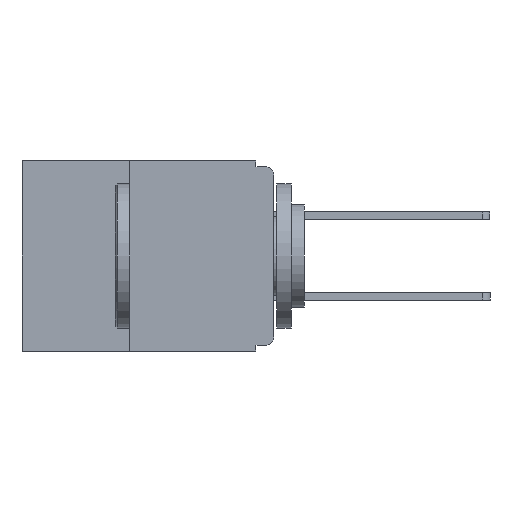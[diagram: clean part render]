
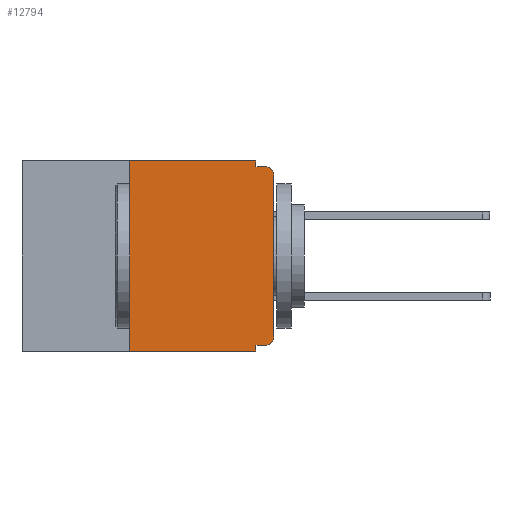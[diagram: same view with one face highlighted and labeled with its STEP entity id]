
A CAD part, left-side view. The second image highlights one B-rep face of the part: STEP entity #12794.
In plain terms, the highlighted planar face has unit normal (-1, 0, 0).
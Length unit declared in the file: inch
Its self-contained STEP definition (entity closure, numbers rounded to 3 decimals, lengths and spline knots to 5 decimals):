
#298 = DIRECTION ( 'NONE',  ( 0., 1., 0. ) ) ;
#384 = DIRECTION ( 'NONE',  ( 0., 0., -1. ) ) ;
#423 = ORIENTED_EDGE ( 'NONE', *, *, #16707, .F. ) ;
#598 = CARTESIAN_POINT ( 'NONE',  ( 0., 0.25, -0.33 ) ) ;
#791 = DIRECTION ( 'NONE',  ( 0., 0., 1. ) ) ;
#1061 = LINE ( 'NONE', #6859, #5854 ) ;
#1530 = ORIENTED_EDGE ( 'NONE', *, *, #5502, .F. ) ;
#1548 = EDGE_CURVE ( 'NONE', #3851, #9073, #20003, .T. ) ;
#1618 = DIRECTION ( 'NONE',  ( 0., 0., 1. ) ) ;
#1698 = CARTESIAN_POINT ( 'NONE',  ( 0., 0.031, 0. ) ) ;
#2040 = CARTESIAN_POINT ( 'NONE',  ( 0., 0., -0.32 ) ) ;
#2406 = ORIENTED_EDGE ( 'NONE', *, *, #16976, .F. ) ;
#2468 = EDGE_CURVE ( 'NONE', #5348, #15666, #21885, .T. ) ;
#3175 = CARTESIAN_POINT ( 'NONE',  ( 0., 0.25, 0. ) ) ;
#3291 = VERTEX_POINT ( 'NONE', #16460 ) ;
#3694 = LINE ( 'NONE', #22372, #10378 ) ;
#3746 = DIRECTION ( 'NONE',  ( 0., -1., 0. ) ) ;
#3851 = VERTEX_POINT ( 'NONE', #5782 ) ;
#3961 = EDGE_CURVE ( 'NONE', #15666, #5482, #3694, .T. ) ;
#4403 = CARTESIAN_POINT ( 'NONE',  ( 0., 0.015, -0.025 ) ) ;
#4457 = LINE ( 'NONE', #15519, #17992 ) ;
#4884 = EDGE_CURVE ( 'NONE', #3291, #14059, #13873, .T. ) ;
#4890 = ORIENTED_EDGE ( 'NONE', *, *, #1548, .T. ) ;
#4951 = DIRECTION ( 'NONE',  ( 0., 0., -1. ) ) ;
#5183 = ORIENTED_EDGE ( 'NONE', *, *, #2468, .F. ) ;
#5348 = VERTEX_POINT ( 'NONE', #13063 ) ;
#5482 = VERTEX_POINT ( 'NONE', #7385 ) ;
#5502 = EDGE_CURVE ( 'NONE', #14059, #5348, #1061, .T. ) ;
#5782 = CARTESIAN_POINT ( 'NONE',  ( 0., 0., -0.305 ) ) ;
#5854 = VECTOR ( 'NONE', #6908, 39.37008 ) ;
#5918 = EDGE_CURVE ( 'NONE', #17478, #3851, #20400, .T. ) ;
#6221 = DIRECTION ( 'NONE',  ( 0., 0., -1. ) ) ;
#6545 = VECTOR ( 'NONE', #1618, 39.37008 ) ;
#6859 = CARTESIAN_POINT ( 'NONE',  ( 0., 0.437, 0. ) ) ;
#6885 = ORIENTED_EDGE ( 'NONE', *, *, #4884, .F. ) ;
#6908 = DIRECTION ( 'NONE',  ( 0., -1., 0. ) ) ;
#7280 = VECTOR ( 'NONE', #298, 39.37008 ) ;
#7385 = CARTESIAN_POINT ( 'NONE',  ( 0., 0.015, -0.01 ) ) ;
#8467 = LINE ( 'NONE', #14328, #17801 ) ;
#8469 = DIRECTION ( 'NONE',  ( 0., 0., -1. ) ) ;
#9073 = VERTEX_POINT ( 'NONE', #19768 ) ;
#9863 = AXIS2_PLACEMENT_3D ( 'NONE', #20633, #18973, #8469 ) ;
#9920 = EDGE_LOOP ( 'NONE', ( #4890, #15395, #18150, #5183, #1530, #6885, #22184, #423, #2406, #12957 ) ) ;
#10378 = VECTOR ( 'NONE', #22081, 39.37008 ) ;
#10852 = EDGE_CURVE ( 'NONE', #3291, #18784, #8467, .T. ) ;
#12794 = ADVANCED_FACE ( 'NONE', ( #21772 ), #22323, .F. ) ;
#12957 = ORIENTED_EDGE ( 'NONE', *, *, #5918, .T. ) ;
#13063 = CARTESIAN_POINT ( 'NONE',  ( 0., 0.031, 0. ) ) ;
#13873 = LINE ( 'NONE', #598, #18002 ) ;
#14059 = VERTEX_POINT ( 'NONE', #3175 ) ;
#14172 = CARTESIAN_POINT ( 'NONE',  ( 0., 0.031, -0.01 ) ) ;
#14328 = CARTESIAN_POINT ( 'NONE',  ( 0., 0.437, -0.33 ) ) ;
#14999 = VERTEX_POINT ( 'NONE', #19332 ) ;
#15395 = ORIENTED_EDGE ( 'NONE', *, *, #21621, .T. ) ;
#15429 = DIRECTION ( 'NONE',  ( 0., 0., -1. ) ) ;
#15458 = CARTESIAN_POINT ( 'NONE',  ( 0., 0.015, -0.305 ) ) ;
#15476 = DIRECTION ( 'NONE',  ( -1., 0., 0. ) ) ;
#15519 = CARTESIAN_POINT ( 'NONE',  ( 0., 0.031, -0.33 ) ) ;
#15623 = AXIS2_PLACEMENT_3D ( 'NONE', #15458, #15476, #15429 ) ;
#15666 = VERTEX_POINT ( 'NONE', #14172 ) ;
#16460 = CARTESIAN_POINT ( 'NONE',  ( 0., 0.25, -0.33 ) ) ;
#16606 = LINE ( 'NONE', #2040, #7280 ) ;
#16707 = EDGE_CURVE ( 'NONE', #14999, #18784, #4457, .T. ) ;
#16761 = DIRECTION ( 'NONE',  ( -1., 0., 0. ) ) ;
#16976 = EDGE_CURVE ( 'NONE', #17478, #14999, #16606, .T. ) ;
#17297 = VECTOR ( 'NONE', #384, 39.37008 ) ;
#17478 = VERTEX_POINT ( 'NONE', #18414 ) ;
#17801 = VECTOR ( 'NONE', #3746, 39.37008 ) ;
#17992 = VECTOR ( 'NONE', #4951, 39.37008 ) ;
#18002 = VECTOR ( 'NONE', #791, 39.37008 ) ;
#18150 = ORIENTED_EDGE ( 'NONE', *, *, #3961, .F. ) ;
#18414 = CARTESIAN_POINT ( 'NONE',  ( 0., 0.015, -0.32 ) ) ;
#18784 = VERTEX_POINT ( 'NONE', #22023 ) ;
#18973 = DIRECTION ( 'NONE',  ( 1., 0., 0. ) ) ;
#19332 = CARTESIAN_POINT ( 'NONE',  ( 0., 0.031, -0.32 ) ) ;
#19398 = AXIS2_PLACEMENT_3D ( 'NONE', #4403, #16761, #6221 ) ;
#19768 = CARTESIAN_POINT ( 'NONE',  ( 0., 0., -0.025 ) ) ;
#19773 = CARTESIAN_POINT ( 'NONE',  ( 0., 0., 0. ) ) ;
#20003 = LINE ( 'NONE', #19773, #6545 ) ;
#20400 = CIRCLE ( 'NONE', #15623, 0.015 ) ;
#20633 = CARTESIAN_POINT ( 'NONE',  ( 0., 0.437, 0. ) ) ;
#21621 = EDGE_CURVE ( 'NONE', #9073, #5482, #21835, .T. ) ;
#21772 = FACE_OUTER_BOUND ( 'NONE', #9920, .T. ) ;
#21835 = CIRCLE ( 'NONE', #19398, 0.015 ) ;
#21885 = LINE ( 'NONE', #1698, #17297 ) ;
#22023 = CARTESIAN_POINT ( 'NONE',  ( 0., 0.031, -0.33 ) ) ;
#22081 = DIRECTION ( 'NONE',  ( 0., -1., 0. ) ) ;
#22184 = ORIENTED_EDGE ( 'NONE', *, *, #10852, .T. ) ;
#22323 = PLANE ( 'NONE',  #9863 ) ;
#22372 = CARTESIAN_POINT ( 'NONE',  ( 0., 0., -0.01 ) ) ;
